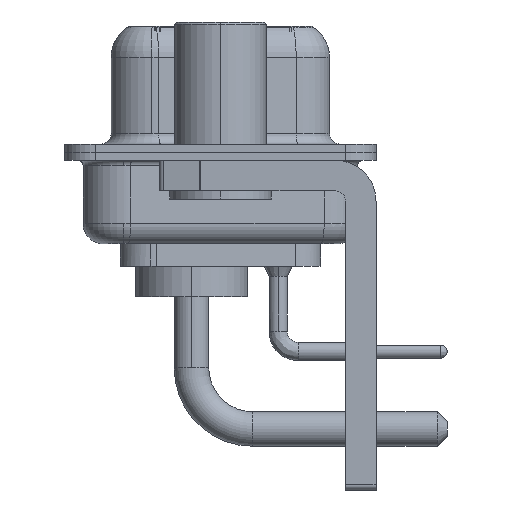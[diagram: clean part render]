
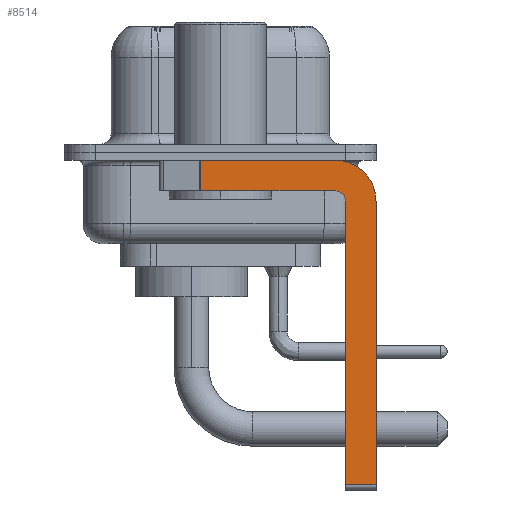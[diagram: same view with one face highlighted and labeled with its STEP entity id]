
A CAD part, left-side view. The second image highlights one B-rep face of the part: STEP entity #8514.
In plain terms, the highlighted planar face has unit normal (-1, 0, 0).
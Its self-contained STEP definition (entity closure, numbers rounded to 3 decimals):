
#45 = CARTESIAN_POINT ( 'NONE',  ( -2.9, 0.978, -1.9 ) ) ;
#625 = CARTESIAN_POINT ( 'NONE',  ( -2.9, -5.65, -16.35 ) ) ;
#627 = CARTESIAN_POINT ( 'NONE',  ( -2.9, -5.65, -2.4 ) ) ;
#982 = ORIENTED_EDGE ( 'NONE', *, *, #11004, .F. ) ;
#1317 = VECTOR ( 'NONE', #12899, 1000. ) ;
#1953 = VERTEX_POINT ( 'NONE', #8468 ) ;
#1981 = CARTESIAN_POINT ( 'NONE',  ( -2.9, -5.65, -1.9 ) ) ;
#2246 = EDGE_CURVE ( 'NONE', #7261, #9959, #22490, .T. ) ;
#2709 = VECTOR ( 'NONE', #13118, 1000. ) ;
#3087 = VERTEX_POINT ( 'NONE', #12727 ) ;
#3508 = ORIENTED_EDGE ( 'NONE', *, *, #9247, .F. ) ;
#3525 = DIRECTION ( 'NONE',  ( -1., 0., 0. ) ) ;
#3569 = LINE ( 'NONE', #3685, #11596 ) ;
#3639 = EDGE_CURVE ( 'NONE', #1953, #11976, #19773, .T. ) ;
#3685 = CARTESIAN_POINT ( 'NONE',  ( -2.9, -7.65, -2.4 ) ) ;
#3697 = CARTESIAN_POINT ( 'NONE',  ( -2.9, -5.65, -1.9 ) ) ;
#4145 = DIRECTION ( 'NONE',  ( 0., 1., 0. ) ) ;
#4359 = FACE_OUTER_BOUND ( 'NONE', #19020, .T. ) ;
#4564 = VERTEX_POINT ( 'NONE', #3697 ) ;
#4973 = VECTOR ( 'NONE', #4145, 1000. ) ;
#5294 = ORIENTED_EDGE ( 'NONE', *, *, #14162, .F. ) ;
#5540 = DIRECTION ( 'NONE',  ( 0., 0., 1. ) ) ;
#5790 = LINE ( 'NONE', #45, #2709 ) ;
#5803 = DIRECTION ( 'NONE',  ( 0., 0., -1. ) ) ;
#5849 = ORIENTED_EDGE ( 'NONE', *, *, #22554, .T. ) ;
#6230 = CARTESIAN_POINT ( 'NONE',  ( -2.9, -7.65, -2.4 ) ) ;
#6513 = DIRECTION ( 'NONE',  ( 0., 0., -1. ) ) ;
#6534 = EDGE_CURVE ( 'NONE', #11976, #9669, #3569, .T. ) ;
#6682 = CARTESIAN_POINT ( 'NONE',  ( -2.9, -6.15, -16.35 ) ) ;
#7261 = VERTEX_POINT ( 'NONE', #6682 ) ;
#7708 = CIRCLE ( 'NONE', #9266, 0.5 ) ;
#8316 = DIRECTION ( 'NONE',  ( 1., 0., 0. ) ) ;
#8468 = CARTESIAN_POINT ( 'NONE',  ( -2.9, -5.65, -0.4 ) ) ;
#8514 = ADVANCED_FACE ( 'NONE', ( #4359 ), #21160, .F. ) ;
#9247 = EDGE_CURVE ( 'NONE', #22100, #1953, #18084, .T. ) ;
#9266 = AXIS2_PLACEMENT_3D ( 'NONE', #19968, #3525, #5540 ) ;
#9430 = LINE ( 'NONE', #1981, #4973 ) ;
#9648 = CARTESIAN_POINT ( 'NONE',  ( -2.9, -6.15, -16.6 ) ) ;
#9669 = VERTEX_POINT ( 'NONE', #13940 ) ;
#9763 = LINE ( 'NONE', #625, #15605 ) ;
#9959 = VERTEX_POINT ( 'NONE', #19551 ) ;
#10759 = DIRECTION ( 'NONE',  ( 0., -1., 0. ) ) ;
#11004 = EDGE_CURVE ( 'NONE', #4564, #3087, #9430, .T. ) ;
#11432 = EDGE_CURVE ( 'NONE', #22100, #3087, #5790, .T. ) ;
#11596 = VECTOR ( 'NONE', #12441, 1000. ) ;
#11976 = VERTEX_POINT ( 'NONE', #6230 ) ;
#12441 = DIRECTION ( 'NONE',  ( 0., 0., -1. ) ) ;
#12727 = CARTESIAN_POINT ( 'NONE',  ( -2.9, 0.978, -1.9 ) ) ;
#12899 = DIRECTION ( 'NONE',  ( 0., 0., 1. ) ) ;
#13118 = DIRECTION ( 'NONE',  ( 0., 0., -1. ) ) ;
#13940 = CARTESIAN_POINT ( 'NONE',  ( -2.9, -7.65, -16.35 ) ) ;
#14162 = EDGE_CURVE ( 'NONE', #9959, #4564, #7708, .T. ) ;
#15274 = ORIENTED_EDGE ( 'NONE', *, *, #2246, .F. ) ;
#15605 = VECTOR ( 'NONE', #22622, 1000. ) ;
#15655 = CARTESIAN_POINT ( 'NONE',  ( -2.9, 0.978, -0.4 ) ) ;
#16652 = ORIENTED_EDGE ( 'NONE', *, *, #6534, .F. ) ;
#17441 = CARTESIAN_POINT ( 'NONE',  ( -2.9, -5.65, -2.4 ) ) ;
#18084 = LINE ( 'NONE', #21314, #19852 ) ;
#19020 = EDGE_LOOP ( 'NONE', ( #3508, #20858, #982, #5294, #15274, #5849, #16652, #23276 ) ) ;
#19551 = CARTESIAN_POINT ( 'NONE',  ( -2.9, -6.15, -2.4 ) ) ;
#19773 = CIRCLE ( 'NONE', #22861, 2. ) ;
#19852 = VECTOR ( 'NONE', #10759, 1000. ) ;
#19968 = CARTESIAN_POINT ( 'NONE',  ( -2.9, -5.65, -2.4 ) ) ;
#20569 = DIRECTION ( 'NONE',  ( 1., 0., 0. ) ) ;
#20858 = ORIENTED_EDGE ( 'NONE', *, *, #11432, .T. ) ;
#21160 = PLANE ( 'NONE',  #21890 ) ;
#21314 = CARTESIAN_POINT ( 'NONE',  ( -2.9, 3., -0.4 ) ) ;
#21890 = AXIS2_PLACEMENT_3D ( 'NONE', #17441, #8316, #6513 ) ;
#22100 = VERTEX_POINT ( 'NONE', #15655 ) ;
#22490 = LINE ( 'NONE', #9648, #1317 ) ;
#22554 = EDGE_CURVE ( 'NONE', #7261, #9669, #9763, .T. ) ;
#22622 = DIRECTION ( 'NONE',  ( 0., -1., 0. ) ) ;
#22861 = AXIS2_PLACEMENT_3D ( 'NONE', #627, #20569, #5803 ) ;
#23276 = ORIENTED_EDGE ( 'NONE', *, *, #3639, .F. ) ;
